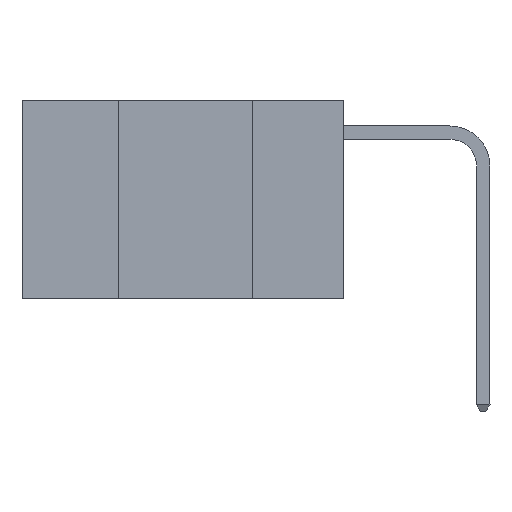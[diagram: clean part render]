
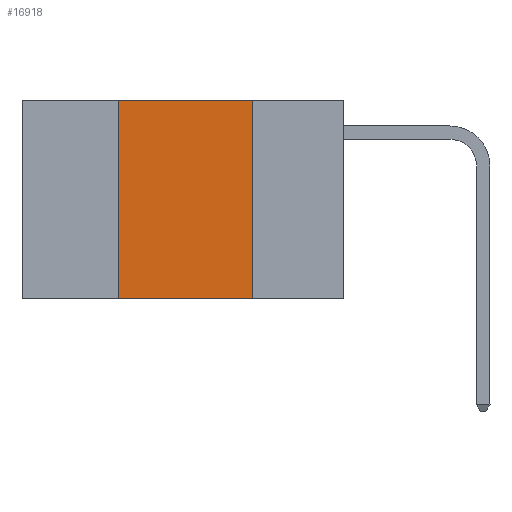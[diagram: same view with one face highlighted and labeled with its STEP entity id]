
A CAD part, left-side view. The second image highlights one B-rep face of the part: STEP entity #16918.
In plain terms, the highlighted planar face has unit normal (-1, 0, 0).
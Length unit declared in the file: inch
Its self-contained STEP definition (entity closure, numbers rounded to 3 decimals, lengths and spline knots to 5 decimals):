
#1212 = DIRECTION ( 'NONE',  ( 0., 0., -1. ) ) ;
#1288 = VECTOR ( 'NONE', #5077, 39.37008 ) ;
#2607 = ORIENTED_EDGE ( 'NONE', *, *, #12659, .F. ) ;
#2615 = CARTESIAN_POINT ( 'NONE',  ( 0., 0.6, 0. ) ) ;
#2757 = DIRECTION ( 'NONE',  ( 1., 0., 0. ) ) ;
#2837 = LINE ( 'NONE', #14361, #7513 ) ;
#3807 = CARTESIAN_POINT ( 'NONE',  ( 0., 0.6, 0. ) ) ;
#3928 = VERTEX_POINT ( 'NONE', #4905 ) ;
#3944 = CARTESIAN_POINT ( 'NONE',  ( 0., 0.17, 0. ) ) ;
#4905 = CARTESIAN_POINT ( 'NONE',  ( 0., 0.17, -0.37 ) ) ;
#5077 = DIRECTION ( 'NONE',  ( 0., -1., 0. ) ) ;
#5515 = ORIENTED_EDGE ( 'NONE', *, *, #24120, .T. ) ;
#5823 = DIRECTION ( 'NONE',  ( 0., 0., -1. ) ) ;
#6330 = CARTESIAN_POINT ( 'NONE',  ( 0., 0.17, 0. ) ) ;
#7513 = VECTOR ( 'NONE', #16505, 39.37008 ) ;
#9003 = LINE ( 'NONE', #24428, #1288 ) ;
#9391 = LINE ( 'NONE', #3807, #12898 ) ;
#10145 = EDGE_LOOP ( 'NONE', ( #2607, #21755, #15619, #5515 ) ) ;
#10356 = PLANE ( 'NONE',  #23332 ) ;
#10711 = VECTOR ( 'NONE', #5823, 39.37008 ) ;
#11621 = VERTEX_POINT ( 'NONE', #3944 ) ;
#12659 = EDGE_CURVE ( 'NONE', #11621, #3928, #13653, .T. ) ;
#12898 = VECTOR ( 'NONE', #18916, 39.37008 ) ;
#13653 = LINE ( 'NONE', #6330, #10711 ) ;
#14361 = CARTESIAN_POINT ( 'NONE',  ( 0., 0.42, 0. ) ) ;
#14730 = VERTEX_POINT ( 'NONE', #24386 ) ;
#14955 = EDGE_CURVE ( 'NONE', #24245, #14730, #2837, .T. ) ;
#15619 = ORIENTED_EDGE ( 'NONE', *, *, #14955, .F. ) ;
#16425 = FACE_OUTER_BOUND ( 'NONE', #10145, .T. ) ;
#16505 = DIRECTION ( 'NONE',  ( 0., 0., 1. ) ) ;
#16918 = ADVANCED_FACE ( 'NONE', ( #16425 ), #10356, .F. ) ;
#18916 = DIRECTION ( 'NONE',  ( 0., -1., 0. ) ) ;
#20379 = EDGE_CURVE ( 'NONE', #14730, #11621, #9391, .T. ) ;
#21755 = ORIENTED_EDGE ( 'NONE', *, *, #20379, .F. ) ;
#23332 = AXIS2_PLACEMENT_3D ( 'NONE', #2615, #2757, #1212 ) ;
#24120 = EDGE_CURVE ( 'NONE', #24245, #3928, #9003, .T. ) ;
#24245 = VERTEX_POINT ( 'NONE', #24812 ) ;
#24386 = CARTESIAN_POINT ( 'NONE',  ( 0., 0.42, 0. ) ) ;
#24428 = CARTESIAN_POINT ( 'NONE',  ( 0., 0.6, -0.37 ) ) ;
#24812 = CARTESIAN_POINT ( 'NONE',  ( 0., 0.42, -0.37 ) ) ;
